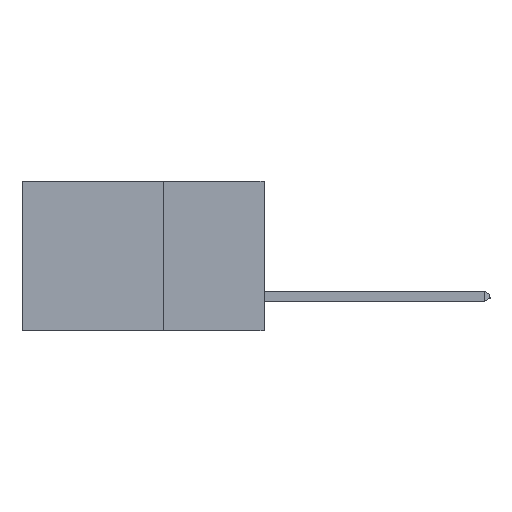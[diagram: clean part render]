
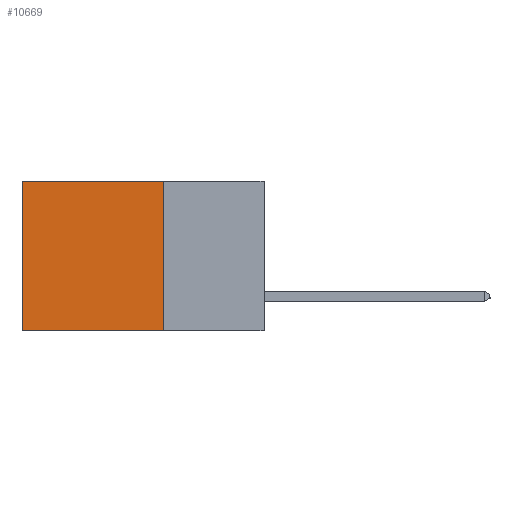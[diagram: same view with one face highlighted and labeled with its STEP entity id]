
A CAD part, left-side view. The second image highlights one B-rep face of the part: STEP entity #10669.
In plain terms, the highlighted planar face has unit normal (-1, 0, 0).
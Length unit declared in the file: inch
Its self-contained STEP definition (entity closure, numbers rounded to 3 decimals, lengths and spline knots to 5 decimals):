
#319 = VERTEX_POINT ( 'NONE', #1594 ) ;
#420 = VECTOR ( 'NONE', #3584, 39.37008 ) ;
#620 = DIRECTION ( 'NONE',  ( 0., 1., 0. ) ) ;
#714 = CARTESIAN_POINT ( 'NONE',  ( 0.298, 0.25, -0.37 ) ) ;
#1132 = DIRECTION ( 'NONE',  ( 0., 1., 0. ) ) ;
#1398 = ORIENTED_EDGE ( 'NONE', *, *, #5865, .T. ) ;
#1594 = CARTESIAN_POINT ( 'NONE',  ( 0.298, 0.25, 0. ) ) ;
#2153 = EDGE_CURVE ( 'NONE', #4645, #7600, #5180, .T. ) ;
#2698 = DIRECTION ( 'NONE',  ( 0., 0., -1. ) ) ;
#2900 = FACE_OUTER_BOUND ( 'NONE', #7081, .T. ) ;
#3439 = VECTOR ( 'NONE', #1132, 39.37008 ) ;
#3584 = DIRECTION ( 'NONE',  ( 0., 0., -1. ) ) ;
#3810 = VECTOR ( 'NONE', #2698, 39.37008 ) ;
#3951 = CARTESIAN_POINT ( 'NONE',  ( 0.298, 0.25, -0.37 ) ) ;
#4269 = CARTESIAN_POINT ( 'NONE',  ( 0.298, 0.6, -0.37 ) ) ;
#4426 = EDGE_CURVE ( 'NONE', #8371, #7600, #8791, .T. ) ;
#4645 = VERTEX_POINT ( 'NONE', #10616 ) ;
#5163 = DIRECTION ( 'NONE',  ( 1., 0., 0. ) ) ;
#5180 = LINE ( 'NONE', #10223, #420 ) ;
#5610 = ORIENTED_EDGE ( 'NONE', *, *, #7742, .F. ) ;
#5865 = EDGE_CURVE ( 'NONE', #319, #4645, #8265, .T. ) ;
#6661 = VECTOR ( 'NONE', #620, 39.37008 ) ;
#7081 = EDGE_LOOP ( 'NONE', ( #9465, #10686, #5610, #1398 ) ) ;
#7422 = CARTESIAN_POINT ( 'NONE',  ( 0.298, 0.25, 0. ) ) ;
#7600 = VERTEX_POINT ( 'NONE', #4269 ) ;
#7692 = PLANE ( 'NONE',  #8904 ) ;
#7742 = EDGE_CURVE ( 'NONE', #319, #8371, #8358, .T. ) ;
#8265 = LINE ( 'NONE', #7422, #3439 ) ;
#8358 = LINE ( 'NONE', #10948, #3810 ) ;
#8371 = VERTEX_POINT ( 'NONE', #3951 ) ;
#8791 = LINE ( 'NONE', #714, #6661 ) ;
#8904 = AXIS2_PLACEMENT_3D ( 'NONE', #10065, #5163, #10829 ) ;
#9465 = ORIENTED_EDGE ( 'NONE', *, *, #2153, .T. ) ;
#10065 = CARTESIAN_POINT ( 'NONE',  ( 0.298, 0.25, 0. ) ) ;
#10223 = CARTESIAN_POINT ( 'NONE',  ( 0.298, 0.6, 0. ) ) ;
#10616 = CARTESIAN_POINT ( 'NONE',  ( 0.298, 0.6, 0. ) ) ;
#10669 = ADVANCED_FACE ( 'NONE', ( #2900 ), #7692, .F. ) ;
#10686 = ORIENTED_EDGE ( 'NONE', *, *, #4426, .F. ) ;
#10829 = DIRECTION ( 'NONE',  ( 0., 0., -1. ) ) ;
#10948 = CARTESIAN_POINT ( 'NONE',  ( 0.298, 0.25, 0. ) ) ;
